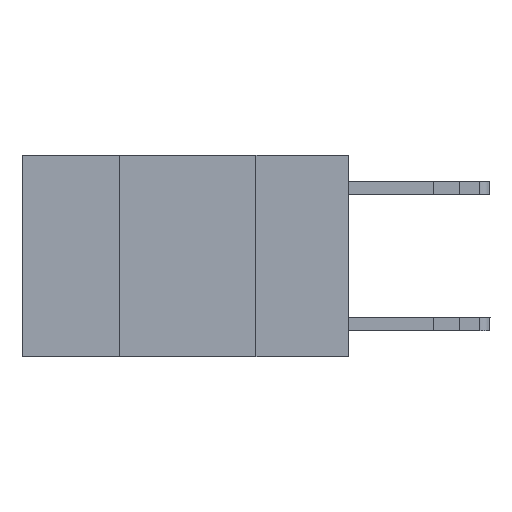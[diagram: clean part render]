
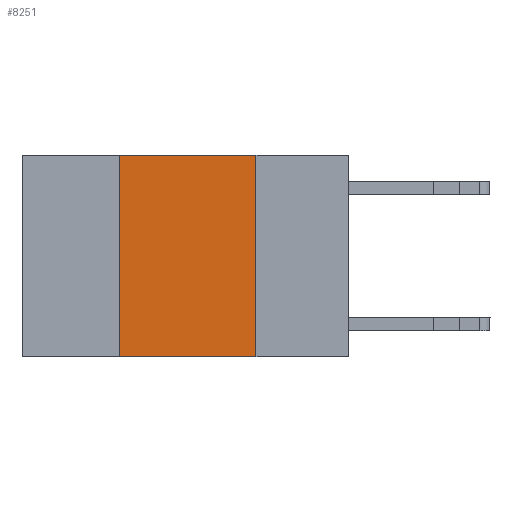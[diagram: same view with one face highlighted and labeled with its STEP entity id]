
A CAD part, left-side view. The second image highlights one B-rep face of the part: STEP entity #8251.
In plain terms, the highlighted planar face has unit normal (-1, 0, 0).
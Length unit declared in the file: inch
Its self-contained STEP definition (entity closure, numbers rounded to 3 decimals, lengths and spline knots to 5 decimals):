
#197 = VECTOR ( 'NONE', #11383, 39.37008 ) ;
#569 = ORIENTED_EDGE ( 'NONE', *, *, #13371, .F. ) ;
#1094 = DIRECTION ( 'NONE',  ( 0., 0., 1. ) ) ;
#1142 = CARTESIAN_POINT ( 'NONE',  ( 0., 0.17, 0. ) ) ;
#1417 = VECTOR ( 'NONE', #13488, 39.37008 ) ;
#1593 = VECTOR ( 'NONE', #14960, 39.37008 ) ;
#4181 = CARTESIAN_POINT ( 'NONE',  ( 0., 0.6, 0. ) ) ;
#4273 = CARTESIAN_POINT ( 'NONE',  ( 0., 0.17, 0. ) ) ;
#4870 = VERTEX_POINT ( 'NONE', #7655 ) ;
#5503 = LINE ( 'NONE', #4181, #1417 ) ;
#5863 = EDGE_LOOP ( 'NONE', ( #11304, #569, #8296, #15118 ) ) ;
#6209 = LINE ( 'NONE', #14176, #197 ) ;
#6376 = VERTEX_POINT ( 'NONE', #10379 ) ;
#7655 = CARTESIAN_POINT ( 'NONE',  ( 0., 0.42, 0. ) ) ;
#7703 = DIRECTION ( 'NONE',  ( 1., 0., 0. ) ) ;
#8012 = LINE ( 'NONE', #13379, #14149 ) ;
#8251 = ADVANCED_FACE ( 'NONE', ( #15596 ), #16886, .F. ) ;
#8296 = ORIENTED_EDGE ( 'NONE', *, *, #16257, .F. ) ;
#10201 = AXIS2_PLACEMENT_3D ( 'NONE', #15507, #7703, #14451 ) ;
#10218 = EDGE_CURVE ( 'NONE', #15407, #6376, #16270, .T. ) ;
#10379 = CARTESIAN_POINT ( 'NONE',  ( 0., 0.17, -0.37 ) ) ;
#11304 = ORIENTED_EDGE ( 'NONE', *, *, #10218, .F. ) ;
#11383 = DIRECTION ( 'NONE',  ( 0., -1., 0. ) ) ;
#11942 = CARTESIAN_POINT ( 'NONE',  ( 0., 0.42, -0.37 ) ) ;
#13371 = EDGE_CURVE ( 'NONE', #4870, #15407, #5503, .T. ) ;
#13379 = CARTESIAN_POINT ( 'NONE',  ( 0., 0.42, 0. ) ) ;
#13488 = DIRECTION ( 'NONE',  ( 0., -1., 0. ) ) ;
#14149 = VECTOR ( 'NONE', #1094, 39.37008 ) ;
#14176 = CARTESIAN_POINT ( 'NONE',  ( 0., 0.6, -0.37 ) ) ;
#14451 = DIRECTION ( 'NONE',  ( 0., 0., -1. ) ) ;
#14960 = DIRECTION ( 'NONE',  ( 0., 0., -1. ) ) ;
#15118 = ORIENTED_EDGE ( 'NONE', *, *, #15730, .T. ) ;
#15407 = VERTEX_POINT ( 'NONE', #1142 ) ;
#15507 = CARTESIAN_POINT ( 'NONE',  ( 0., 0.6, 0. ) ) ;
#15596 = FACE_OUTER_BOUND ( 'NONE', #5863, .T. ) ;
#15730 = EDGE_CURVE ( 'NONE', #16319, #6376, #6209, .T. ) ;
#16257 = EDGE_CURVE ( 'NONE', #16319, #4870, #8012, .T. ) ;
#16270 = LINE ( 'NONE', #4273, #1593 ) ;
#16319 = VERTEX_POINT ( 'NONE', #11942 ) ;
#16886 = PLANE ( 'NONE',  #10201 ) ;
